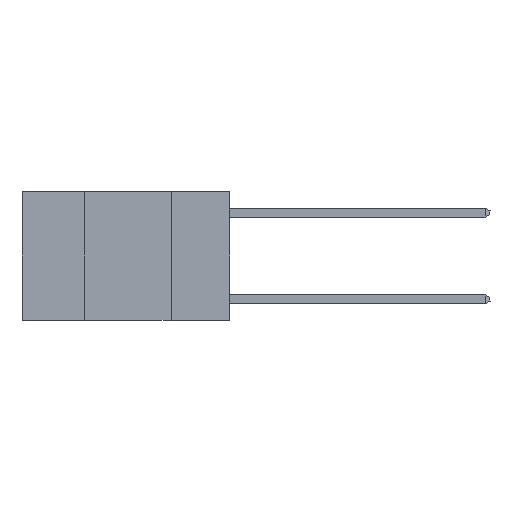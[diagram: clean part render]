
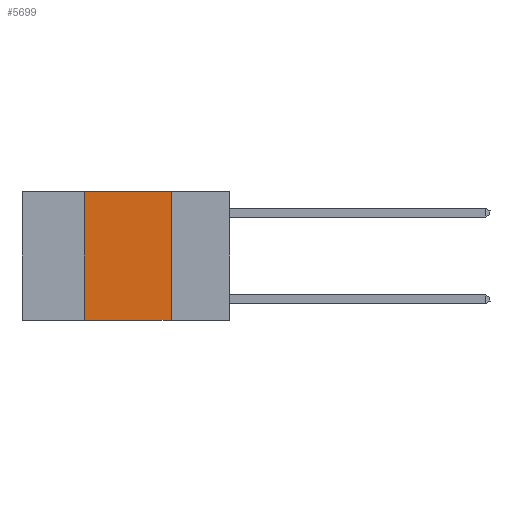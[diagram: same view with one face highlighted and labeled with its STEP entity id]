
A CAD part, left-side view. The second image highlights one B-rep face of the part: STEP entity #5699.
In plain terms, the highlighted planar face has unit normal (-1, 0, 0).
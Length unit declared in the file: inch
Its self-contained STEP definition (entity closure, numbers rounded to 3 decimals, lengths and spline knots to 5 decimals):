
#15 = LINE ( 'NONE', #11042, #16409 ) ;
#852 = VECTOR ( 'NONE', #17776, 39.37008 ) ;
#1465 = DIRECTION ( 'NONE',  ( 0., 0., 1. ) ) ;
#1961 = CARTESIAN_POINT ( 'NONE',  ( 0., 0.42, 0. ) ) ;
#2817 = CARTESIAN_POINT ( 'NONE',  ( 0., 0.17, 0. ) ) ;
#3360 = CARTESIAN_POINT ( 'NONE',  ( 0., 0.6, -0.37 ) ) ;
#4917 = ORIENTED_EDGE ( 'NONE', *, *, #20271, .F. ) ;
#5292 = CARTESIAN_POINT ( 'NONE',  ( 0., 0.17, 0. ) ) ;
#5699 = ADVANCED_FACE ( 'NONE', ( #6410 ), #16030, .F. ) ;
#6410 = FACE_OUTER_BOUND ( 'NONE', #8878, .T. ) ;
#6432 = VERTEX_POINT ( 'NONE', #1961 ) ;
#6734 = DIRECTION ( 'NONE',  ( 0., 0., -1. ) ) ;
#7300 = LINE ( 'NONE', #3360, #14217 ) ;
#7857 = DIRECTION ( 'NONE',  ( 0., -1., 0. ) ) ;
#8461 = CARTESIAN_POINT ( 'NONE',  ( 0., 0.42, -0.37 ) ) ;
#8709 = ORIENTED_EDGE ( 'NONE', *, *, #8979, .F. ) ;
#8861 = AXIS2_PLACEMENT_3D ( 'NONE', #19056, #16097, #6734 ) ;
#8878 = EDGE_LOOP ( 'NONE', ( #8709, #16940, #4917, #17876 ) ) ;
#8979 = EDGE_CURVE ( 'NONE', #10876, #9276, #13641, .T. ) ;
#9276 = VERTEX_POINT ( 'NONE', #18428 ) ;
#10876 = VERTEX_POINT ( 'NONE', #2817 ) ;
#10950 = LINE ( 'NONE', #12719, #19501 ) ;
#11042 = CARTESIAN_POINT ( 'NONE',  ( 0., 0.6, 0. ) ) ;
#12719 = CARTESIAN_POINT ( 'NONE',  ( 0., 0.42, 0. ) ) ;
#13641 = LINE ( 'NONE', #5292, #852 ) ;
#13933 = EDGE_CURVE ( 'NONE', #18723, #9276, #7300, .T. ) ;
#14217 = VECTOR ( 'NONE', #19043, 39.37008 ) ;
#16030 = PLANE ( 'NONE',  #8861 ) ;
#16097 = DIRECTION ( 'NONE',  ( 1., 0., 0. ) ) ;
#16409 = VECTOR ( 'NONE', #7857, 39.37008 ) ;
#16940 = ORIENTED_EDGE ( 'NONE', *, *, #17738, .F. ) ;
#17738 = EDGE_CURVE ( 'NONE', #6432, #10876, #15, .T. ) ;
#17776 = DIRECTION ( 'NONE',  ( 0., 0., -1. ) ) ;
#17876 = ORIENTED_EDGE ( 'NONE', *, *, #13933, .T. ) ;
#18428 = CARTESIAN_POINT ( 'NONE',  ( 0., 0.17, -0.37 ) ) ;
#18723 = VERTEX_POINT ( 'NONE', #8461 ) ;
#19043 = DIRECTION ( 'NONE',  ( 0., -1., 0. ) ) ;
#19056 = CARTESIAN_POINT ( 'NONE',  ( 0., 0.6, 0. ) ) ;
#19501 = VECTOR ( 'NONE', #1465, 39.37008 ) ;
#20271 = EDGE_CURVE ( 'NONE', #18723, #6432, #10950, .T. ) ;
